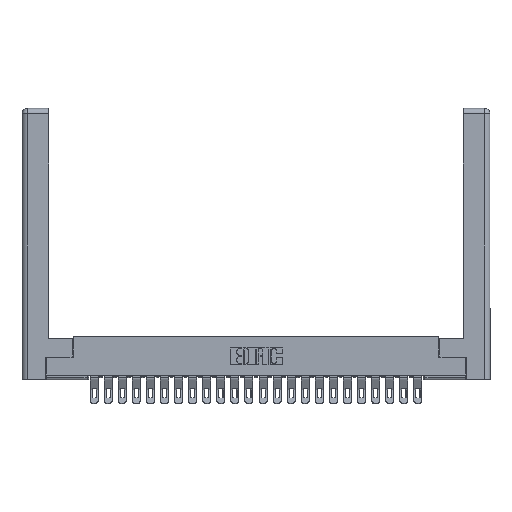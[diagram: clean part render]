
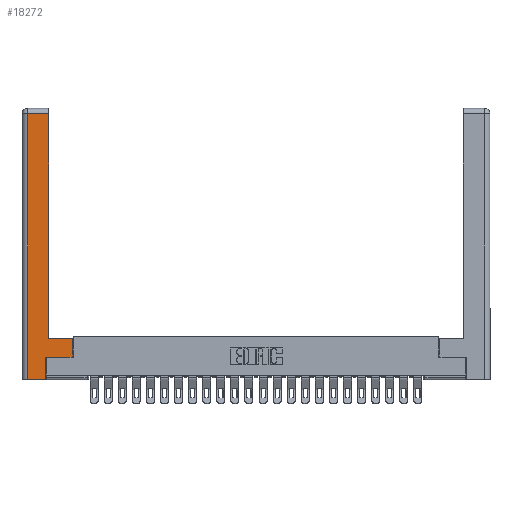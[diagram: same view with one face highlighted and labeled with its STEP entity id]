
A CAD part, top view. The second image highlights one B-rep face of the part: STEP entity #18272.
In plain terms, the highlighted planar face has unit normal (0, 0, 1).
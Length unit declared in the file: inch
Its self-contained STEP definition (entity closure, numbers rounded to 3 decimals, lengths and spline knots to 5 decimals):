
#487 = ORIENTED_EDGE ( 'NONE', *, *, #25430, .T. ) ;
#880 = CARTESIAN_POINT ( 'NONE',  ( 0.565, 0.245, 0. ) ) ;
#1234 = AXIS2_PLACEMENT_3D ( 'NONE', #18245, #7956, #16230 ) ;
#1417 = LINE ( 'NONE', #12223, #26681 ) ;
#1438 = EDGE_LOOP ( 'NONE', ( #4679, #6545, #487, #5572, #11529, #3703, #3943, #13947 ) ) ;
#1693 = DIRECTION ( 'NONE',  ( 0., 1., 0. ) ) ;
#1749 = FACE_OUTER_BOUND ( 'NONE', #1438, .T. ) ;
#2553 = DIRECTION ( 'NONE',  ( 0., 1., 0. ) ) ;
#2618 = VERTEX_POINT ( 'NONE', #20790 ) ;
#2745 = VERTEX_POINT ( 'NONE', #26547 ) ;
#3273 = VECTOR ( 'NONE', #15856, 39.37008 ) ;
#3703 = ORIENTED_EDGE ( 'NONE', *, *, #25447, .T. ) ;
#3943 = ORIENTED_EDGE ( 'NONE', *, *, #4249, .T. ) ;
#4010 = CARTESIAN_POINT ( 'NONE',  ( 0.265, 0., 0. ) ) ;
#4249 = EDGE_CURVE ( 'NONE', #2618, #15386, #1417, .T. ) ;
#4679 = ORIENTED_EDGE ( 'NONE', *, *, #17469, .T. ) ;
#4978 = CARTESIAN_POINT ( 'NONE',  ( 0.265, 0.245, 0. ) ) ;
#5316 = CARTESIAN_POINT ( 'NONE',  ( 0.0615, 0., 0. ) ) ;
#5572 = ORIENTED_EDGE ( 'NONE', *, *, #5956, .T. ) ;
#5956 = EDGE_CURVE ( 'NONE', #24879, #16914, #17654, .T. ) ;
#6520 = DIRECTION ( 'NONE',  ( 0., 1., 0. ) ) ;
#6545 = ORIENTED_EDGE ( 'NONE', *, *, #17811, .T. ) ;
#7344 = CARTESIAN_POINT ( 'NONE',  ( 0.265, 0., 0. ) ) ;
#7583 = CARTESIAN_POINT ( 'NONE',  ( 0.295, 0.45, 0. ) ) ;
#7932 = VECTOR ( 'NONE', #13577, 39.37008 ) ;
#7956 = DIRECTION ( 'NONE',  ( 0., 0., -1. ) ) ;
#8116 = LINE ( 'NONE', #20715, #10674 ) ;
#8359 = VECTOR ( 'NONE', #21849, 39.37008 ) ;
#8741 = LINE ( 'NONE', #4978, #16270 ) ;
#9980 = PLANE ( 'NONE',  #1234 ) ;
#10197 = VERTEX_POINT ( 'NONE', #25415 ) ;
#10629 = CARTESIAN_POINT ( 'NONE',  ( 0.0615, 0., 0. ) ) ;
#10674 = VECTOR ( 'NONE', #22221, 39.37008 ) ;
#10888 = VERTEX_POINT ( 'NONE', #23878 ) ;
#11288 = LINE ( 'NONE', #880, #7932 ) ;
#11458 = CARTESIAN_POINT ( 'NONE',  ( 0.565, 0.45, 0. ) ) ;
#11529 = ORIENTED_EDGE ( 'NONE', *, *, #16522, .T. ) ;
#11547 = LINE ( 'NONE', #5316, #8359 ) ;
#11569 = VECTOR ( 'NONE', #26171, 39.37008 ) ;
#12223 = CARTESIAN_POINT ( 'NONE',  ( 0.565, 0.45, 0. ) ) ;
#13577 = DIRECTION ( 'NONE',  ( 1., 0., 0. ) ) ;
#13947 = ORIENTED_EDGE ( 'NONE', *, *, #14018, .T. ) ;
#14018 = EDGE_CURVE ( 'NONE', #15386, #10197, #24262, .T. ) ;
#14819 = VERTEX_POINT ( 'NONE', #14948 ) ;
#14925 = LINE ( 'NONE', #16943, #15029 ) ;
#14948 = CARTESIAN_POINT ( 'NONE',  ( 0.265, 0.245, 0. ) ) ;
#15029 = VECTOR ( 'NONE', #6520, 39.37008 ) ;
#15386 = VERTEX_POINT ( 'NONE', #11458 ) ;
#15856 = DIRECTION ( 'NONE',  ( -1., 0., 0. ) ) ;
#16230 = DIRECTION ( 'NONE',  ( -1., 0., 0. ) ) ;
#16270 = VECTOR ( 'NONE', #2553, 39.37008 ) ;
#16522 = EDGE_CURVE ( 'NONE', #16914, #14819, #8741, .T. ) ;
#16914 = VERTEX_POINT ( 'NONE', #4010 ) ;
#16943 = CARTESIAN_POINT ( 'NONE',  ( 0.295, 3., 0. ) ) ;
#17469 = EDGE_CURVE ( 'NONE', #10197, #10888, #14925, .T. ) ;
#17654 = LINE ( 'NONE', #7344, #11569 ) ;
#17811 = EDGE_CURVE ( 'NONE', #10888, #2745, #8116, .T. ) ;
#18245 = CARTESIAN_POINT ( 'NONE',  ( 0., 0., 0. ) ) ;
#18272 = ADVANCED_FACE ( 'NONE', ( #1749 ), #9980, .F. ) ;
#20715 = CARTESIAN_POINT ( 'NONE',  ( 0.0615, 2.94, 0. ) ) ;
#20790 = CARTESIAN_POINT ( 'NONE',  ( 0.565, 0.245, 0. ) ) ;
#21849 = DIRECTION ( 'NONE',  ( 0., -1., 0. ) ) ;
#22221 = DIRECTION ( 'NONE',  ( -1., 0., 0. ) ) ;
#23878 = CARTESIAN_POINT ( 'NONE',  ( 0.295, 2.94, 0. ) ) ;
#24262 = LINE ( 'NONE', #7583, #3273 ) ;
#24879 = VERTEX_POINT ( 'NONE', #10629 ) ;
#25415 = CARTESIAN_POINT ( 'NONE',  ( 0.295, 0.45, 0. ) ) ;
#25430 = EDGE_CURVE ( 'NONE', #2745, #24879, #11547, .T. ) ;
#25447 = EDGE_CURVE ( 'NONE', #14819, #2618, #11288, .T. ) ;
#26171 = DIRECTION ( 'NONE',  ( 1., 0., 0. ) ) ;
#26547 = CARTESIAN_POINT ( 'NONE',  ( 0.0615, 2.94, 0. ) ) ;
#26681 = VECTOR ( 'NONE', #1693, 39.37008 ) ;
